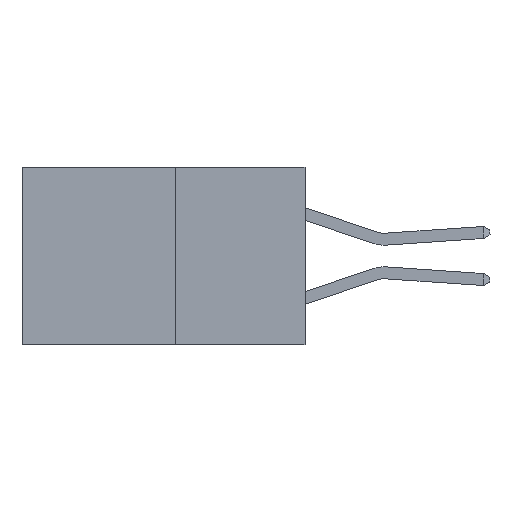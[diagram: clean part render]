
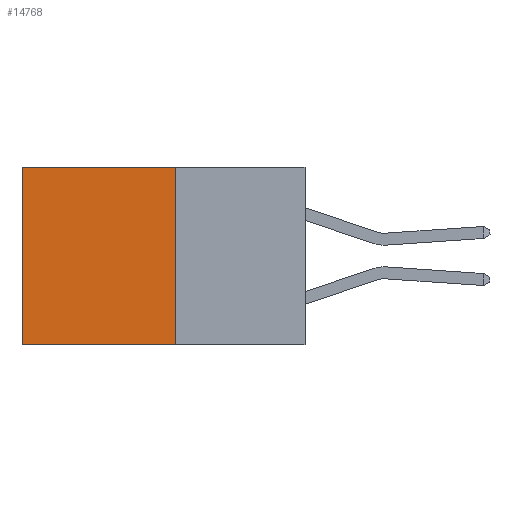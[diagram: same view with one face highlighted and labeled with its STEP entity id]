
A CAD part, left-side view. The second image highlights one B-rep face of the part: STEP entity #14768.
In plain terms, the highlighted planar face has unit normal (-1, 0, 0).
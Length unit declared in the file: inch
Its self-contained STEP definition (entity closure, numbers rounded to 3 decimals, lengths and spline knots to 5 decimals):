
#499 = DIRECTION ( 'NONE',  ( 0., 0., -1. ) ) ;
#726 = AXIS2_PLACEMENT_3D ( 'NONE', #16678, #10316, #499 ) ;
#1818 = CARTESIAN_POINT ( 'NONE',  ( 0.277, 0.27, -0.37 ) ) ;
#1837 = CARTESIAN_POINT ( 'NONE',  ( 0.277, 0.27, -0.37 ) ) ;
#2028 = DIRECTION ( 'NONE',  ( 0., 1., 0. ) ) ;
#2049 = VERTEX_POINT ( 'NONE', #13705 ) ;
#3219 = VECTOR ( 'NONE', #11599, 39.37008 ) ;
#6785 = CARTESIAN_POINT ( 'NONE',  ( 0.277, 0.27, -0.37 ) ) ;
#7014 = CARTESIAN_POINT ( 'NONE',  ( 0.277, 0.27, 0. ) ) ;
#8162 = CARTESIAN_POINT ( 'NONE',  ( 0.277, 0.59, 0. ) ) ;
#8706 = CARTESIAN_POINT ( 'NONE',  ( 0.277, 0.59, -0.37 ) ) ;
#8712 = PLANE ( 'NONE',  #726 ) ;
#8965 = VERTEX_POINT ( 'NONE', #6785 ) ;
#9407 = ORIENTED_EDGE ( 'NONE', *, *, #10441, .F. ) ;
#9894 = ORIENTED_EDGE ( 'NONE', *, *, #18888, .T. ) ;
#9916 = LINE ( 'NONE', #8706, #18868 ) ;
#10107 = DIRECTION ( 'NONE',  ( 0., 0., -1. ) ) ;
#10316 = DIRECTION ( 'NONE',  ( 1., 0., 0. ) ) ;
#10441 = EDGE_CURVE ( 'NONE', #17010, #8965, #14157, .T. ) ;
#10722 = VECTOR ( 'NONE', #2028, 39.37008 ) ;
#11599 = DIRECTION ( 'NONE',  ( 0., 1., 0. ) ) ;
#11873 = LINE ( 'NONE', #1837, #3219 ) ;
#13705 = CARTESIAN_POINT ( 'NONE',  ( 0.277, 0.59, -0.37 ) ) ;
#13970 = FACE_OUTER_BOUND ( 'NONE', #14177, .T. ) ;
#14157 = LINE ( 'NONE', #1818, #17865 ) ;
#14177 = EDGE_LOOP ( 'NONE', ( #9894, #17910, #9407, #15694 ) ) ;
#14709 = EDGE_CURVE ( 'NONE', #17010, #20477, #14988, .T. ) ;
#14768 = ADVANCED_FACE ( 'NONE', ( #13970 ), #8712, .F. ) ;
#14988 = LINE ( 'NONE', #18114, #10722 ) ;
#15694 = ORIENTED_EDGE ( 'NONE', *, *, #14709, .T. ) ;
#16678 = CARTESIAN_POINT ( 'NONE',  ( 0.277, 0.27, -0.37 ) ) ;
#17010 = VERTEX_POINT ( 'NONE', #7014 ) ;
#17865 = VECTOR ( 'NONE', #10107, 39.37008 ) ;
#17910 = ORIENTED_EDGE ( 'NONE', *, *, #19965, .F. ) ;
#18114 = CARTESIAN_POINT ( 'NONE',  ( 0.277, 0.27, 0. ) ) ;
#18868 = VECTOR ( 'NONE', #19816, 39.37008 ) ;
#18888 = EDGE_CURVE ( 'NONE', #20477, #2049, #9916, .T. ) ;
#19816 = DIRECTION ( 'NONE',  ( 0., 0., -1. ) ) ;
#19965 = EDGE_CURVE ( 'NONE', #8965, #2049, #11873, .T. ) ;
#20477 = VERTEX_POINT ( 'NONE', #8162 ) ;
